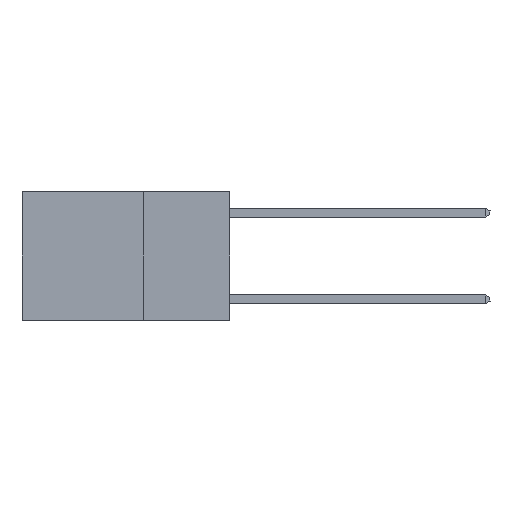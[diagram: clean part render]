
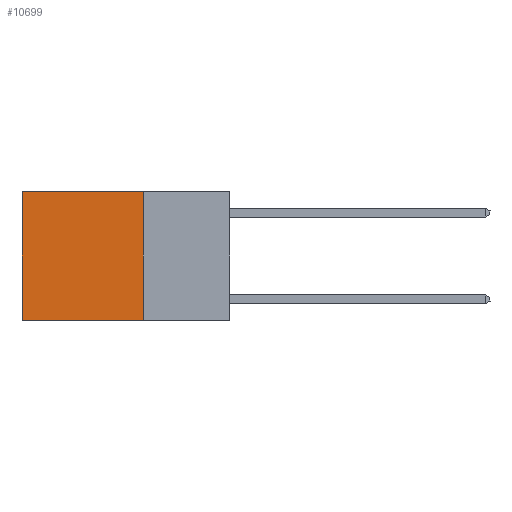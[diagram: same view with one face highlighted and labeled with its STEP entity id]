
A CAD part, left-side view. The second image highlights one B-rep face of the part: STEP entity #10699.
In plain terms, the highlighted planar face has unit normal (-1, 0, 0).
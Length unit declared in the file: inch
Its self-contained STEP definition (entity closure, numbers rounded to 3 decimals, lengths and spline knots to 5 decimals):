
#284 = CARTESIAN_POINT ( 'NONE',  ( 0.2625, 0.6, -0.37 ) ) ;
#566 = ORIENTED_EDGE ( 'NONE', *, *, #10423, .T. ) ;
#823 = VERTEX_POINT ( 'NONE', #284 ) ;
#1034 = EDGE_CURVE ( 'NONE', #4702, #14238, #7997, .T. ) ;
#1160 = DIRECTION ( 'NONE',  ( 0., 1., 0. ) ) ;
#1360 = VECTOR ( 'NONE', #5764, 39.37008 ) ;
#1423 = ORIENTED_EDGE ( 'NONE', *, *, #1034, .F. ) ;
#1903 = DIRECTION ( 'NONE',  ( 0., 0., -1. ) ) ;
#1946 = CARTESIAN_POINT ( 'NONE',  ( 0.2625, 0.25, 0. ) ) ;
#2802 = CARTESIAN_POINT ( 'NONE',  ( 0.2625, 0.25, -0.37 ) ) ;
#2941 = DIRECTION ( 'NONE',  ( 0., 1., 0. ) ) ;
#3278 = VERTEX_POINT ( 'NONE', #12872 ) ;
#4149 = LINE ( 'NONE', #14032, #7777 ) ;
#4702 = VERTEX_POINT ( 'NONE', #12798 ) ;
#5097 = VECTOR ( 'NONE', #1160, 39.37008 ) ;
#5764 = DIRECTION ( 'NONE',  ( 0., 0., -1. ) ) ;
#6624 = EDGE_CURVE ( 'NONE', #14238, #823, #13945, .T. ) ;
#6853 = VECTOR ( 'NONE', #2941, 39.37008 ) ;
#7457 = EDGE_LOOP ( 'NONE', ( #14102, #13343, #1423, #566 ) ) ;
#7462 = CARTESIAN_POINT ( 'NONE',  ( 0.2625, 0.25, 0. ) ) ;
#7777 = VECTOR ( 'NONE', #1903, 39.37008 ) ;
#7883 = EDGE_CURVE ( 'NONE', #3278, #823, #4149, .T. ) ;
#7997 = LINE ( 'NONE', #1946, #1360 ) ;
#8150 = PLANE ( 'NONE',  #13114 ) ;
#8313 = DIRECTION ( 'NONE',  ( 1., 0., 0. ) ) ;
#10423 = EDGE_CURVE ( 'NONE', #4702, #3278, #14760, .T. ) ;
#10699 = ADVANCED_FACE ( 'NONE', ( #15448 ), #8150, .F. ) ;
#12225 = CARTESIAN_POINT ( 'NONE',  ( 0.2625, 0.25, -0.37 ) ) ;
#12798 = CARTESIAN_POINT ( 'NONE',  ( 0.2625, 0.25, 0. ) ) ;
#12872 = CARTESIAN_POINT ( 'NONE',  ( 0.2625, 0.6, 0. ) ) ;
#13114 = AXIS2_PLACEMENT_3D ( 'NONE', #15218, #8313, #13121 ) ;
#13121 = DIRECTION ( 'NONE',  ( 0., 0., -1. ) ) ;
#13343 = ORIENTED_EDGE ( 'NONE', *, *, #6624, .F. ) ;
#13945 = LINE ( 'NONE', #2802, #6853 ) ;
#14032 = CARTESIAN_POINT ( 'NONE',  ( 0.2625, 0.6, 0. ) ) ;
#14102 = ORIENTED_EDGE ( 'NONE', *, *, #7883, .T. ) ;
#14238 = VERTEX_POINT ( 'NONE', #12225 ) ;
#14760 = LINE ( 'NONE', #7462, #5097 ) ;
#15218 = CARTESIAN_POINT ( 'NONE',  ( 0.2625, 0.25, 0. ) ) ;
#15448 = FACE_OUTER_BOUND ( 'NONE', #7457, .T. ) ;
